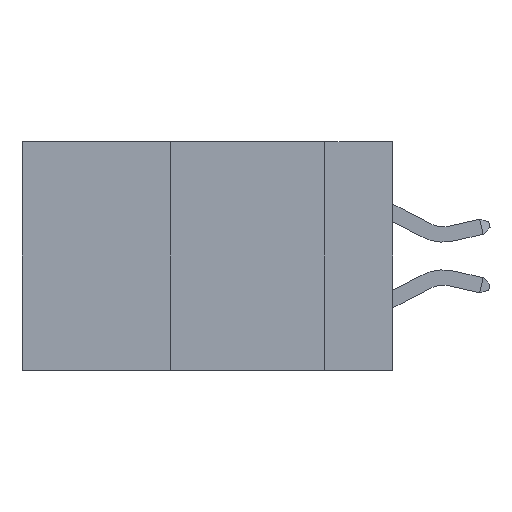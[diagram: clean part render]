
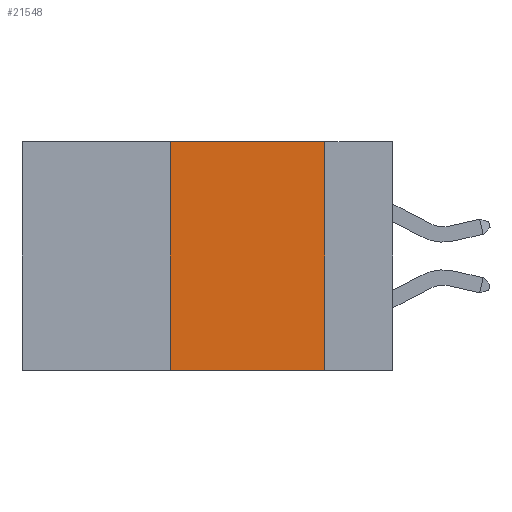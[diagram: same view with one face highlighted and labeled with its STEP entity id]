
A CAD part, left-side view. The second image highlights one B-rep face of the part: STEP entity #21548.
In plain terms, the highlighted planar face has unit normal (-1, 0, 0).
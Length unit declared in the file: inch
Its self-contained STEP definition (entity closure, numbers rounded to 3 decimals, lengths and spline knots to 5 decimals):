
#555 = EDGE_CURVE ( 'NONE', #19866, #16465, #17613, .T. ) ;
#566 = VECTOR ( 'NONE', #17032, 39.37008 ) ;
#619 = CARTESIAN_POINT ( 'NONE',  ( 0., 0.6, 0. ) ) ;
#805 = DIRECTION ( 'NONE',  ( 0., 0., -1. ) ) ;
#1935 = CARTESIAN_POINT ( 'NONE',  ( 0., 0.6, 0. ) ) ;
#2524 = AXIS2_PLACEMENT_3D ( 'NONE', #1935, #13026, #22344 ) ;
#2736 = LINE ( 'NONE', #21182, #3767 ) ;
#2948 = ORIENTED_EDGE ( 'NONE', *, *, #3729, .T. ) ;
#3240 = CARTESIAN_POINT ( 'NONE',  ( 0., 0.11, -0.37 ) ) ;
#3729 = EDGE_CURVE ( 'NONE', #23344, #17931, #12963, .T. ) ;
#3747 = PLANE ( 'NONE',  #2524 ) ;
#3767 = VECTOR ( 'NONE', #4798, 39.37008 ) ;
#4794 = ORIENTED_EDGE ( 'NONE', *, *, #9365, .F. ) ;
#4798 = DIRECTION ( 'NONE',  ( 0., 0., 1. ) ) ;
#6357 = DIRECTION ( 'NONE',  ( 0., -1., 0. ) ) ;
#7678 = CARTESIAN_POINT ( 'NONE',  ( 0., 0.11, 0. ) ) ;
#8488 = LINE ( 'NONE', #13710, #12320 ) ;
#9365 = EDGE_CURVE ( 'NONE', #16465, #17931, #8488, .T. ) ;
#11225 = EDGE_CURVE ( 'NONE', #23344, #19866, #2736, .T. ) ;
#12320 = VECTOR ( 'NONE', #805, 39.37008 ) ;
#12963 = LINE ( 'NONE', #20329, #566 ) ;
#13026 = DIRECTION ( 'NONE',  ( 1., 0., 0. ) ) ;
#13260 = ORIENTED_EDGE ( 'NONE', *, *, #11225, .F. ) ;
#13710 = CARTESIAN_POINT ( 'NONE',  ( 0., 0.11, 0. ) ) ;
#16465 = VERTEX_POINT ( 'NONE', #7678 ) ;
#17032 = DIRECTION ( 'NONE',  ( 0., -1., 0. ) ) ;
#17613 = LINE ( 'NONE', #619, #18729 ) ;
#17931 = VERTEX_POINT ( 'NONE', #3240 ) ;
#18478 = ORIENTED_EDGE ( 'NONE', *, *, #555, .F. ) ;
#18729 = VECTOR ( 'NONE', #6357, 39.37008 ) ;
#19376 = EDGE_LOOP ( 'NONE', ( #4794, #18478, #13260, #2948 ) ) ;
#19866 = VERTEX_POINT ( 'NONE', #21151 ) ;
#20329 = CARTESIAN_POINT ( 'NONE',  ( 0., 0.6, -0.37 ) ) ;
#21151 = CARTESIAN_POINT ( 'NONE',  ( 0., 0.36, 0. ) ) ;
#21182 = CARTESIAN_POINT ( 'NONE',  ( 0., 0.36, 0. ) ) ;
#21548 = ADVANCED_FACE ( 'NONE', ( #21970 ), #3747, .F. ) ;
#21970 = FACE_OUTER_BOUND ( 'NONE', #19376, .T. ) ;
#22195 = CARTESIAN_POINT ( 'NONE',  ( 0., 0.36, -0.37 ) ) ;
#22344 = DIRECTION ( 'NONE',  ( 0., 0., -1. ) ) ;
#23344 = VERTEX_POINT ( 'NONE', #22195 ) ;
